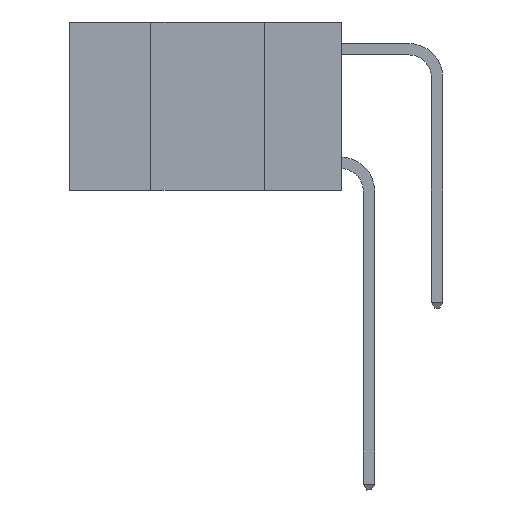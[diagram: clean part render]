
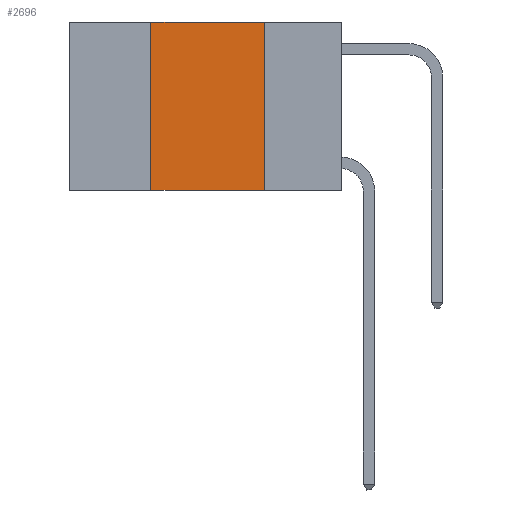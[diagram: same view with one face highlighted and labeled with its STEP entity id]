
A CAD part, left-side view. The second image highlights one B-rep face of the part: STEP entity #2696.
In plain terms, the highlighted planar face has unit normal (-1, 0, 0).
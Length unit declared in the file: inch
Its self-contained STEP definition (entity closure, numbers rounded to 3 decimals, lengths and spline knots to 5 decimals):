
#474 = VERTEX_POINT ( 'NONE', #15121 ) ;
#678 = DIRECTION ( 'NONE',  ( 0., 0., 1. ) ) ;
#1028 = AXIS2_PLACEMENT_3D ( 'NONE', #8549, #12179, #8462 ) ;
#1461 = ORIENTED_EDGE ( 'NONE', *, *, #4055, .F. ) ;
#1836 = VERTEX_POINT ( 'NONE', #14533 ) ;
#1966 = ORIENTED_EDGE ( 'NONE', *, *, #7039, .F. ) ;
#2696 = ADVANCED_FACE ( 'NONE', ( #8372 ), #14783, .F. ) ;
#3206 = LINE ( 'NONE', #12479, #9024 ) ;
#3886 = CARTESIAN_POINT ( 'NONE',  ( 0., 0.42, -0.37 ) ) ;
#4055 = EDGE_CURVE ( 'NONE', #474, #7518, #13873, .T. ) ;
#4337 = DIRECTION ( 'NONE',  ( 0., -1., 0. ) ) ;
#4465 = DIRECTION ( 'NONE',  ( 0., -1., 0. ) ) ;
#4798 = DIRECTION ( 'NONE',  ( 0., 0., -1. ) ) ;
#5617 = EDGE_LOOP ( 'NONE', ( #1461, #1966, #11325, #9824 ) ) ;
#6527 = CARTESIAN_POINT ( 'NONE',  ( 0., 0.17, -0.37 ) ) ;
#6986 = CARTESIAN_POINT ( 'NONE',  ( 0., 0.6, -0.37 ) ) ;
#7039 = EDGE_CURVE ( 'NONE', #1836, #474, #3206, .T. ) ;
#7518 = VERTEX_POINT ( 'NONE', #6527 ) ;
#8372 = FACE_OUTER_BOUND ( 'NONE', #5617, .T. ) ;
#8462 = DIRECTION ( 'NONE',  ( 0., 0., -1. ) ) ;
#8509 = VECTOR ( 'NONE', #4337, 39.37008 ) ;
#8549 = CARTESIAN_POINT ( 'NONE',  ( 0., 0.6, 0. ) ) ;
#9024 = VECTOR ( 'NONE', #4465, 39.37008 ) ;
#9824 = ORIENTED_EDGE ( 'NONE', *, *, #9894, .T. ) ;
#9894 = EDGE_CURVE ( 'NONE', #16520, #7518, #16142, .T. ) ;
#11076 = LINE ( 'NONE', #12406, #16040 ) ;
#11325 = ORIENTED_EDGE ( 'NONE', *, *, #13870, .F. ) ;
#12179 = DIRECTION ( 'NONE',  ( 1., 0., 0. ) ) ;
#12242 = VECTOR ( 'NONE', #4798, 39.37008 ) ;
#12406 = CARTESIAN_POINT ( 'NONE',  ( 0., 0.42, 0. ) ) ;
#12479 = CARTESIAN_POINT ( 'NONE',  ( 0., 0.6, 0. ) ) ;
#13870 = EDGE_CURVE ( 'NONE', #16520, #1836, #11076, .T. ) ;
#13873 = LINE ( 'NONE', #14215, #12242 ) ;
#14215 = CARTESIAN_POINT ( 'NONE',  ( 0., 0.17, 0. ) ) ;
#14533 = CARTESIAN_POINT ( 'NONE',  ( 0., 0.42, 0. ) ) ;
#14783 = PLANE ( 'NONE',  #1028 ) ;
#15121 = CARTESIAN_POINT ( 'NONE',  ( 0., 0.17, 0. ) ) ;
#16040 = VECTOR ( 'NONE', #678, 39.37008 ) ;
#16142 = LINE ( 'NONE', #6986, #8509 ) ;
#16520 = VERTEX_POINT ( 'NONE', #3886 ) ;
